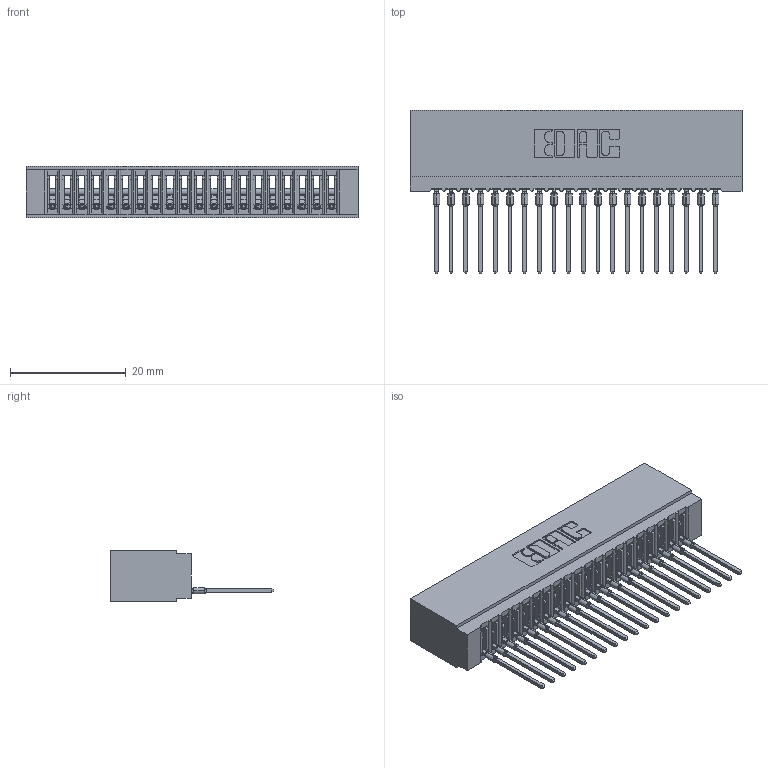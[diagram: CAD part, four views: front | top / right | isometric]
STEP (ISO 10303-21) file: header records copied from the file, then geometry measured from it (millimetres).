
FILE_DESCRIPTION (( 'STEP AP203' ), '1' );
FILE_NAME ('725-020-540-101.STEP', '2026-03-05T21:14:40', ( '' ), ( '' ), 'SwSTEP 2.0', 'SolidWorks 2023', '' );
FILE_SCHEMA (( 'CONFIG_CONTROL_DESIGN' ));
Length unit declared in the file: millimetre
Products named in the file (3): 745-292-001_540; 725 Part_Insulator Option - 01; 725-020-540-101
Assembly tree (21 placements, depth 2):
  725-020-540-101
    725 Part_Insulator Option - 01
    745-292-001_540  x20
Bounding box: 57.4 x 28.21 x 8.89 mm (x, y, z)
Volume: 4526.2 mm3; surface area: 8531.3 mm2
Topology: 21 solids, 21 shells, 2335 faces, 6414 edges, 4048 vertices
Faces by surface type: plane 1395, cylinder 420, bspline 400, torus 120
Entity records: 35998 total; most frequent: CARTESIAN_POINT 6843, ORIENTED_EDGE 6254, DIRECTION 5445, EDGE_CURVE 3127, VECTOR 2825, LINE 2825, VERTEX_POINT 1996, AXIS2_PLACEMENT_3D 1310
